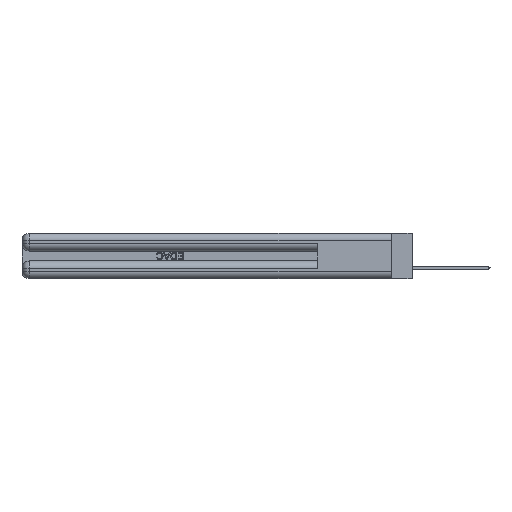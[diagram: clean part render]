
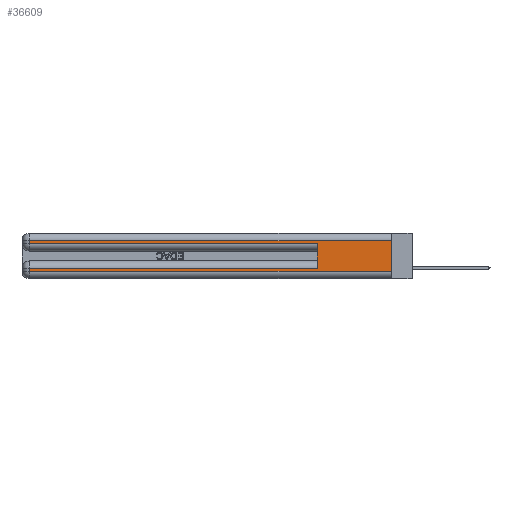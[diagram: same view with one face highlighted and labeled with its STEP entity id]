
A CAD part, left-side view. The second image highlights one B-rep face of the part: STEP entity #36609.
In plain terms, the highlighted planar face has unit normal (-1, 0, 0).
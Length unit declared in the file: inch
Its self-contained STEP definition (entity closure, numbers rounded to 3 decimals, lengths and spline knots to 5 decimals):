
#969 = EDGE_LOOP ( 'NONE', ( #4532, #27146, #18959, #22132, #16416, #40324, #12277, #29723 ) ) ;
#988 = VECTOR ( 'NONE', #27258, 39.37008 ) ;
#1375 = CARTESIAN_POINT ( 'NONE',  ( 0., 2.94, 0.37 ) ) ;
#1967 = LINE ( 'NONE', #25925, #35923 ) ;
#3826 = DIRECTION ( 'NONE',  ( 0., -1., 0. ) ) ;
#4111 = VERTEX_POINT ( 'NONE', #20995 ) ;
#4532 = ORIENTED_EDGE ( 'NONE', *, *, #9214, .F. ) ;
#7895 = LINE ( 'NONE', #34750, #45182 ) ;
#8996 = EDGE_CURVE ( 'NONE', #13293, #4111, #40295, .T. ) ;
#9214 = EDGE_CURVE ( 'NONE', #18472, #37212, #7895, .T. ) ;
#9490 = VECTOR ( 'NONE', #24805, 39.37008 ) ;
#10692 = EDGE_CURVE ( 'NONE', #18472, #22120, #19016, .T. ) ;
#10851 = DIRECTION ( 'NONE',  ( 0., 0., -1. ) ) ;
#11263 = LINE ( 'NONE', #45594, #988 ) ;
#12277 = ORIENTED_EDGE ( 'NONE', *, *, #8996, .T. ) ;
#12591 = AXIS2_PLACEMENT_3D ( 'NONE', #32228, #32799, #32654 ) ;
#13293 = VERTEX_POINT ( 'NONE', #41808 ) ;
#14170 = LINE ( 'NONE', #17175, #18646 ) ;
#15112 = LINE ( 'NONE', #39701, #28185 ) ;
#15179 = CARTESIAN_POINT ( 'NONE',  ( 0., 0., 0.31 ) ) ;
#15340 = VERTEX_POINT ( 'NONE', #33737 ) ;
#15457 = CARTESIAN_POINT ( 'NONE',  ( 0., 0.6, 0.085 ) ) ;
#16126 = CARTESIAN_POINT ( 'NONE',  ( 0., 0.6, 0.145 ) ) ;
#16416 = ORIENTED_EDGE ( 'NONE', *, *, #23265, .F. ) ;
#16550 = CARTESIAN_POINT ( 'NONE',  ( 0., 0.6, 0.285 ) ) ;
#17175 = CARTESIAN_POINT ( 'NONE',  ( 0., 2.94, 0.37 ) ) ;
#18472 = VERTEX_POINT ( 'NONE', #15179 ) ;
#18646 = VECTOR ( 'NONE', #10851, 39.37008 ) ;
#18795 = VECTOR ( 'NONE', #27037, 39.37008 ) ;
#18891 = EDGE_CURVE ( 'NONE', #22120, #15340, #14170, .T. ) ;
#18959 = ORIENTED_EDGE ( 'NONE', *, *, #18891, .T. ) ;
#19016 = LINE ( 'NONE', #46448, #9490 ) ;
#20995 = CARTESIAN_POINT ( 'NONE',  ( 0., 2.94, 0.06 ) ) ;
#21320 = PLANE ( 'NONE',  #12591 ) ;
#22120 = VERTEX_POINT ( 'NONE', #37515 ) ;
#22132 = ORIENTED_EDGE ( 'NONE', *, *, #35607, .T. ) ;
#23265 = EDGE_CURVE ( 'NONE', #31704, #27995, #37351, .T. ) ;
#24805 = DIRECTION ( 'NONE',  ( 0., 1., 0. ) ) ;
#25061 = FACE_OUTER_BOUND ( 'NONE', #969, .T. ) ;
#25925 = CARTESIAN_POINT ( 'NONE',  ( 0., 0., 0.285 ) ) ;
#27037 = DIRECTION ( 'NONE',  ( 0., 0., -1. ) ) ;
#27146 = ORIENTED_EDGE ( 'NONE', *, *, #10692, .T. ) ;
#27258 = DIRECTION ( 'NONE',  ( 0., 1., 0. ) ) ;
#27995 = VERTEX_POINT ( 'NONE', #16550 ) ;
#28185 = VECTOR ( 'NONE', #3826, 39.37008 ) ;
#29723 = ORIENTED_EDGE ( 'NONE', *, *, #45762, .T. ) ;
#31704 = VERTEX_POINT ( 'NONE', #15457 ) ;
#32228 = CARTESIAN_POINT ( 'NONE',  ( 0., 0., 0.37 ) ) ;
#32654 = DIRECTION ( 'NONE',  ( 0., 0., -1. ) ) ;
#32735 = DIRECTION ( 'NONE',  ( 0., -1., 0. ) ) ;
#32799 = DIRECTION ( 'NONE',  ( 1., 0., 0. ) ) ;
#33485 = DIRECTION ( 'NONE',  ( 0., 0., 1. ) ) ;
#33737 = CARTESIAN_POINT ( 'NONE',  ( 0., 2.94, 0.285 ) ) ;
#34750 = CARTESIAN_POINT ( 'NONE',  ( 0., 0., 0.37 ) ) ;
#35607 = EDGE_CURVE ( 'NONE', #15340, #27995, #1967, .T. ) ;
#35751 = VECTOR ( 'NONE', #33485, 39.37008 ) ;
#35923 = VECTOR ( 'NONE', #32735, 39.37008 ) ;
#36609 = ADVANCED_FACE ( 'NONE', ( #25061 ), #21320, .F. ) ;
#37212 = VERTEX_POINT ( 'NONE', #39454 ) ;
#37351 = LINE ( 'NONE', #16126, #35751 ) ;
#37515 = CARTESIAN_POINT ( 'NONE',  ( 0., 2.94, 0.31 ) ) ;
#39454 = CARTESIAN_POINT ( 'NONE',  ( 0., 0., 0.06 ) ) ;
#39701 = CARTESIAN_POINT ( 'NONE',  ( 0., 0., 0.06 ) ) ;
#40295 = LINE ( 'NONE', #1375, #18795 ) ;
#40324 = ORIENTED_EDGE ( 'NONE', *, *, #44973, .T. ) ;
#41808 = CARTESIAN_POINT ( 'NONE',  ( 0., 2.94, 0.085 ) ) ;
#44973 = EDGE_CURVE ( 'NONE', #31704, #13293, #11263, .T. ) ;
#45182 = VECTOR ( 'NONE', #45424, 39.37008 ) ;
#45424 = DIRECTION ( 'NONE',  ( 0., 0., -1. ) ) ;
#45594 = CARTESIAN_POINT ( 'NONE',  ( 0., 0., 0.085 ) ) ;
#45762 = EDGE_CURVE ( 'NONE', #4111, #37212, #15112, .T. ) ;
#46448 = CARTESIAN_POINT ( 'NONE',  ( 0., 0., 0.31 ) ) ;
